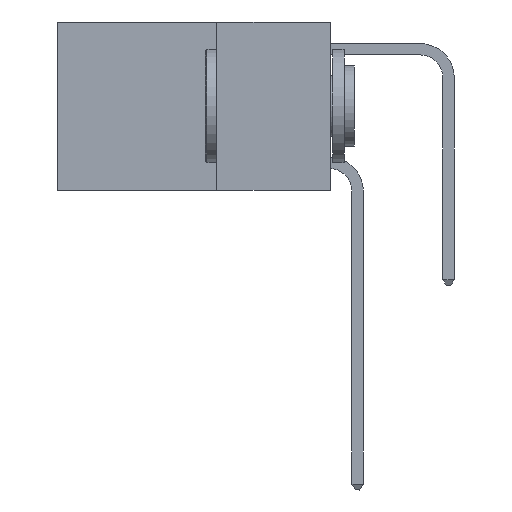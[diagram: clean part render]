
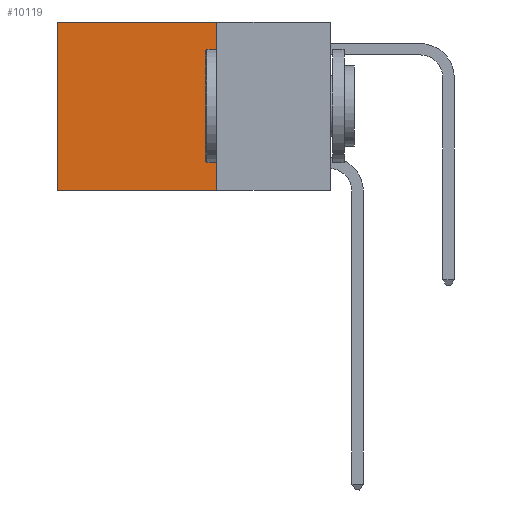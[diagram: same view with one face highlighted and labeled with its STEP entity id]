
A CAD part, left-side view. The second image highlights one B-rep face of the part: STEP entity #10119.
In plain terms, the highlighted planar face has unit normal (-1, 0, 0).
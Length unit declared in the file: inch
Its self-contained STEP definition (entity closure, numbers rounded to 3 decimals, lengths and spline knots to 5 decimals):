
#413 = EDGE_CURVE ( 'NONE', #11443, #9545, #10260, .T. ) ;
#432 = ORIENTED_EDGE ( 'NONE', *, *, #413, .F. ) ;
#475 = VECTOR ( 'NONE', #10990, 39.37008 ) ;
#817 = VERTEX_POINT ( 'NONE', #2307 ) ;
#1221 = PLANE ( 'NONE',  #4994 ) ;
#2137 = EDGE_CURVE ( 'NONE', #817, #11443, #2161, .T. ) ;
#2161 = LINE ( 'NONE', #15495, #16131 ) ;
#2307 = CARTESIAN_POINT ( 'NONE',  ( 0.2625, 0.25, 0. ) ) ;
#2746 = FACE_OUTER_BOUND ( 'NONE', #12195, .T. ) ;
#4939 = DIRECTION ( 'NONE',  ( 1., 0., 0. ) ) ;
#4994 = AXIS2_PLACEMENT_3D ( 'NONE', #14046, #4939, #17684 ) ;
#5175 = ORIENTED_EDGE ( 'NONE', *, *, #15010, .T. ) ;
#5334 = CARTESIAN_POINT ( 'NONE',  ( 0.2625, 0.6, 0. ) ) ;
#5991 = LINE ( 'NONE', #15012, #10313 ) ;
#6322 = DIRECTION ( 'NONE',  ( 0., 0., -1. ) ) ;
#7291 = ORIENTED_EDGE ( 'NONE', *, *, #2137, .F. ) ;
#8282 = EDGE_CURVE ( 'NONE', #817, #20003, #9365, .T. ) ;
#9365 = LINE ( 'NONE', #18218, #22761 ) ;
#9545 = VERTEX_POINT ( 'NONE', #14373 ) ;
#10119 = ADVANCED_FACE ( 'NONE', ( #2746 ), #1221, .F. ) ;
#10260 = LINE ( 'NONE', #10270, #475 ) ;
#10270 = CARTESIAN_POINT ( 'NONE',  ( 0.2625, 0.25, -0.37 ) ) ;
#10313 = VECTOR ( 'NONE', #16826, 39.37008 ) ;
#10912 = DIRECTION ( 'NONE',  ( 0., 1., 0. ) ) ;
#10990 = DIRECTION ( 'NONE',  ( 0., 1., 0. ) ) ;
#11443 = VERTEX_POINT ( 'NONE', #17790 ) ;
#12195 = EDGE_LOOP ( 'NONE', ( #5175, #432, #7291, #20961 ) ) ;
#14046 = CARTESIAN_POINT ( 'NONE',  ( 0.2625, 0.25, 0. ) ) ;
#14373 = CARTESIAN_POINT ( 'NONE',  ( 0.2625, 0.6, -0.37 ) ) ;
#15010 = EDGE_CURVE ( 'NONE', #20003, #9545, #5991, .T. ) ;
#15012 = CARTESIAN_POINT ( 'NONE',  ( 0.2625, 0.6, 0. ) ) ;
#15495 = CARTESIAN_POINT ( 'NONE',  ( 0.2625, 0.25, 0. ) ) ;
#16131 = VECTOR ( 'NONE', #6322, 39.37008 ) ;
#16826 = DIRECTION ( 'NONE',  ( 0., 0., -1. ) ) ;
#17684 = DIRECTION ( 'NONE',  ( 0., 0., -1. ) ) ;
#17790 = CARTESIAN_POINT ( 'NONE',  ( 0.2625, 0.25, -0.37 ) ) ;
#18218 = CARTESIAN_POINT ( 'NONE',  ( 0.2625, 0.25, 0. ) ) ;
#20003 = VERTEX_POINT ( 'NONE', #5334 ) ;
#20961 = ORIENTED_EDGE ( 'NONE', *, *, #8282, .T. ) ;
#22761 = VECTOR ( 'NONE', #10912, 39.37008 ) ;
